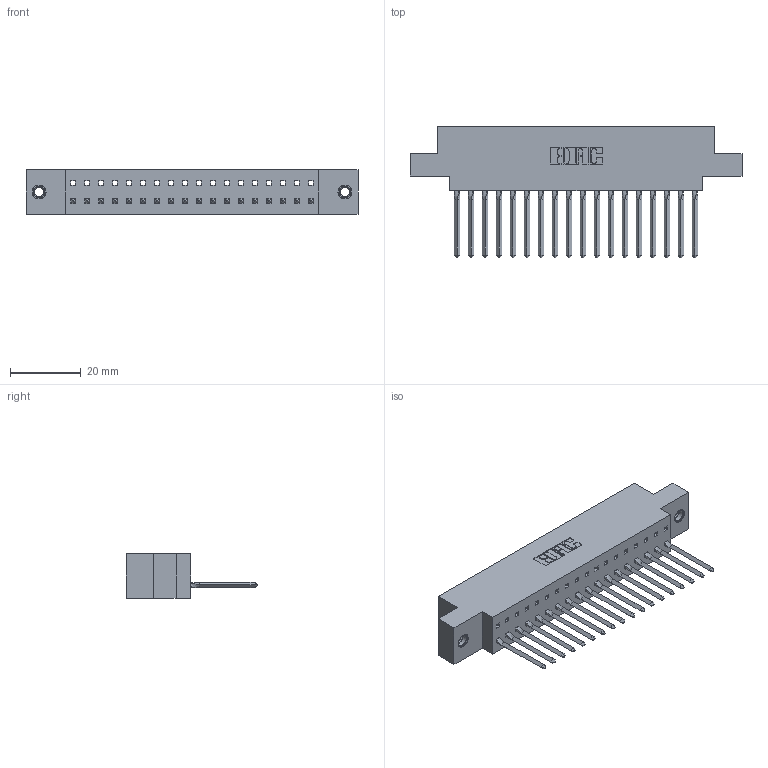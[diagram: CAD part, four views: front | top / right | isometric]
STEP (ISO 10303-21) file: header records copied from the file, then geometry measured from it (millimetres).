
FILE_DESCRIPTION (( 'STEP AP203' ), '1' );
FILE_NAME ('317-018-542-607.STEP', '2020-02-27T15:50:09', ( '' ), ( '' ), 'SwSTEP 2.0', 'SolidWorks 2016', '' );
FILE_SCHEMA (( 'CONFIG_CONTROL_DESIGN' ));
Length unit declared in the file: inch
Products named in the file (4): 317-018-542-607; 317 Part_.156 Dia - TI; 345-250-001_345-250-005-103; 317-290-003_542
Assembly tree (21 placements, depth 2):
  317-018-542-607
    317 Part_.156 Dia - TI
    317-290-003_542  x18
    345-250-001_345-250-005-103  x2
Bounding box: 94.03 x 37.34 x 12.7 mm (x, y, z)
Volume: 13873.6 mm3; surface area: 16422.2 mm2
Topology: 21 solids, 21 shells, 1512 faces, 4317 edges, 2786 vertices
Faces by surface type: plane 1242, cylinder 182, bspline 72, cone 12, torus 4
Entity records: 28994 total; most frequent: CARTESIAN_POINT 5358, ORIENTED_EDGE 5032, DIRECTION 4278, EDGE_CURVE 2516, LINE 2326, VECTOR 2326, VERTEX_POINT 1668, AXIS2_PLACEMENT_3D 976
